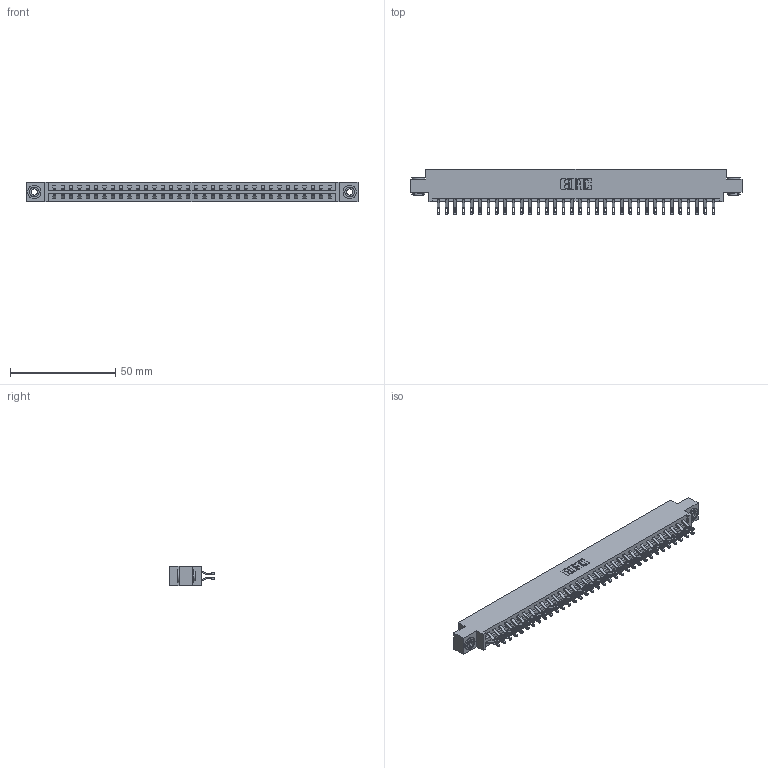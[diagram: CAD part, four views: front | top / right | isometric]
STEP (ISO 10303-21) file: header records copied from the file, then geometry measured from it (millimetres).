
FILE_DESCRIPTION (( 'STEP AP203' ), '1' );
FILE_NAME ('387-068-555-803.STEP', '2019-10-19T21:38:58', ( '' ), ( '' ), 'SwSTEP 2.0', 'SolidWorks 2016', '' );
FILE_SCHEMA (( 'CONFIG_CONTROL_DESIGN' ));
Length unit declared in the file: inch
Products named in the file (4): 337 Part_0.170 Offset - 0.156 Dia-TH; 345-250-002_345-250-002-102; 345-292-001_555 Tail; 387-068-555-803
Assembly tree (71 placements, depth 2):
  387-068-555-803
    337 Part_0.170 Offset - 0.156 Dia-TH
    345-292-001_555 Tail  x68
    345-250-002_345-250-002-102  x2
Bounding box: 157.73 x 21.47 x 9.4 mm (x, y, z)
Volume: 16615.9 mm3; surface area: 19782.1 mm2
Topology: 71 solids, 71 shells, 4236 faces, 13251 edges, 8830 vertices
Faces by surface type: plane 2532, cylinder 1696, cone 8
Entity records: 28504 total; most frequent: CARTESIAN_POINT 4819, ORIENTED_EDGE 4718, DIRECTION 4117, EDGE_CURVE 2359, VECTOR 2187, LINE 2187, VERTEX_POINT 1570, AXIS2_PLACEMENT_3D 965
